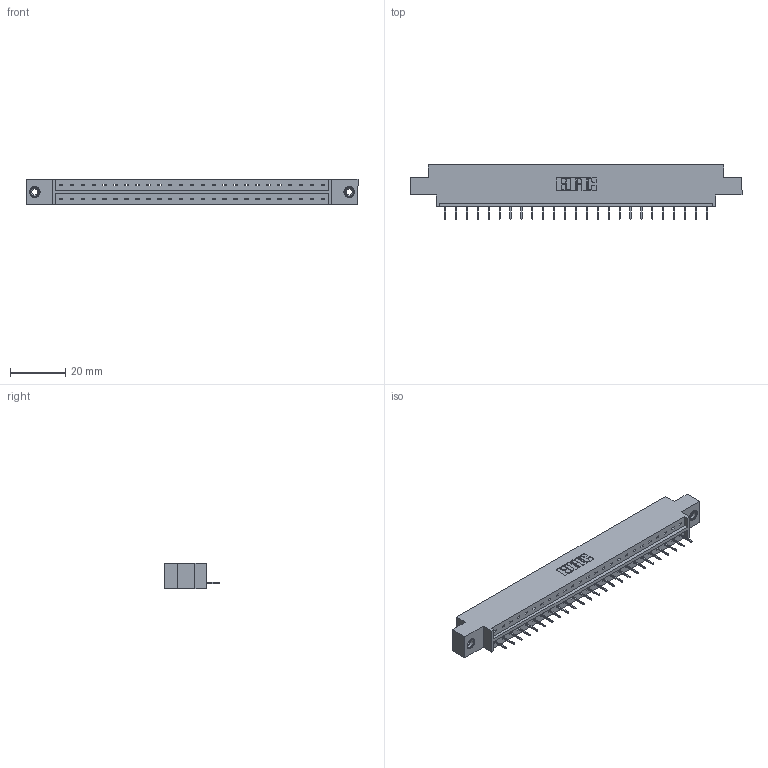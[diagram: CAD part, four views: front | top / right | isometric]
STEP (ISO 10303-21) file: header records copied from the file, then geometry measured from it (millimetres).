
FILE_DESCRIPTION (( 'STEP AP203' ), '1' );
FILE_NAME ('833-025-524-608.STEP', '2020-06-01T23:34:27', ( '' ), ( '' ), 'SwSTEP 2.0', 'SolidWorks 2020', '' );
FILE_SCHEMA (( 'CONFIG_CONTROL_DESIGN' ));
Length unit declared in the file: inch
Products named in the file (4): 833 Part_Offset - .156 Dia - TI; 345-292-001_345-293-124; 345-250-001_345-250-003-102; 833-025-524-608
Assembly tree (28 placements, depth 2):
  833-025-524-608
    833 Part_Offset - .156 Dia - TI
    345-292-001_345-293-124  x25
    345-250-001_345-250-003-102  x2
Bounding box: 120.6 x 19.69 x 9.4 mm (x, y, z)
Volume: 11656.4 mm3; surface area: 12385.2 mm2
Topology: 28 solids, 28 shells, 1728 faces, 4959 edges, 3198 vertices
Faces by surface type: plane 1306, cylinder 406, cone 12, torus 4
Entity records: 18874 total; most frequent: CARTESIAN_POINT 3240, ORIENTED_EDGE 3194, DIRECTION 2801, EDGE_CURVE 1597, VECTOR 1453, LINE 1453, VERTEX_POINT 1056, AXIS2_PLACEMENT_3D 674
